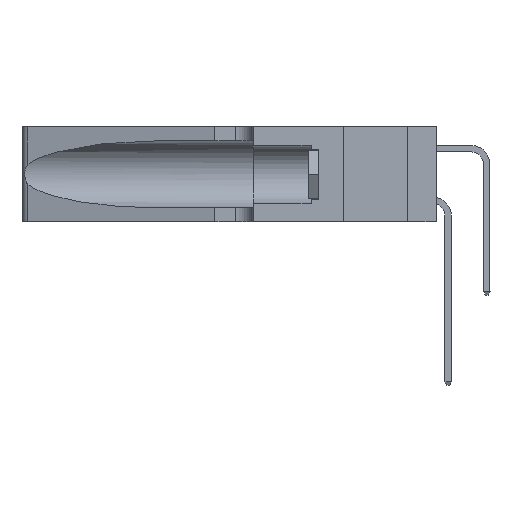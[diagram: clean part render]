
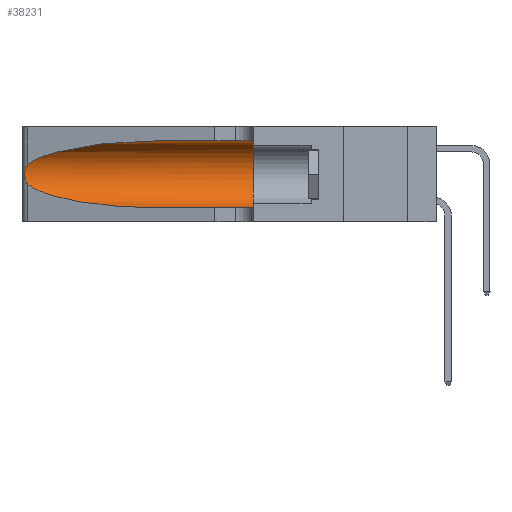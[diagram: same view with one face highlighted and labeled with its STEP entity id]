
A CAD part, left-side view. The second image highlights one B-rep face of the part: STEP entity #38231.
In plain terms, the highlighted cylindrical face has radius 3.308 mm (diameter 6.617 mm), a partial arc.
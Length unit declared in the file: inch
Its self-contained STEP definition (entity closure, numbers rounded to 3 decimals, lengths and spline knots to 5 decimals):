
#231 = CARTESIAN_POINT ( 'NONE',  ( 0.25639, 1.23184, 0.21858 ) ) ;
#267 = CIRCLE ( 'NONE', #12914, 0.13025 ) ;
#367 = CARTESIAN_POINT ( 'NONE',  ( 0.25639, 1.23186, 0.15144 ) ) ;
#790 = CARTESIAN_POINT ( 'NONE',  ( 0.1305, 0.35, 0.05475 ) ) ;
#2662 = CARTESIAN_POINT ( 'NONE',  ( 0.25487, 1.22718, 0.22369 ) ) ;
#3551 = DIRECTION ( 'NONE',  ( 0., -1., 0. ) ) ;
#3570 = CARTESIAN_POINT ( 'NONE',  ( 0.25487, 1.22718, 0.14631 ) ) ;
#3775 = EDGE_CURVE ( 'NONE', #7832, #8609, #11327, .T. ) ;
#4247 =( BOUNDED_CURVE ( )  B_SPLINE_CURVE ( 3, ( #21486, #18471, #12590, #33351 ),
 .UNSPECIFIED., .F., .T. ) 
 B_SPLINE_CURVE_WITH_KNOTS ( ( 4, 4 ),
 ( 1.5708, 2.84003 ),
 .UNSPECIFIED. ) 
 CURVE ( )  GEOMETRIC_REPRESENTATION_ITEM ( )  RATIONAL_B_SPLINE_CURVE ( ( 1., 0.87, 0.87, 1. ) ) 
 REPRESENTATION_ITEM ( '' )  );
#4338 = CARTESIAN_POINT ( 'NONE',  ( 0.1305, 0.72297, 0.31525 ) ) ;
#4430 = EDGE_CURVE ( 'NONE', #9524, #7832, #4247, .T. ) ;
#4561 = VECTOR ( 'NONE', #3551, 39.37008 ) ;
#4654 = EDGE_CURVE ( 'NONE', #17662, #17156, #267, .T. ) ;
#4661 = EDGE_CURVE ( 'NONE', #8609, #13584, #36060, .T. ) ;
#6535 = EDGE_CURVE ( 'NONE', #9524, #17662, #12644, .T. ) ;
#7121 = ORIENTED_EDGE ( 'NONE', *, *, #4430, .T. ) ;
#7679 = CARTESIAN_POINT ( 'NONE',  ( 0.18966, 0.96281, 0.05475 ) ) ;
#7735 = CARTESIAN_POINT ( 'NONE',  ( 0.1305, 1.61858, 0.185 ) ) ;
#7832 = VERTEX_POINT ( 'NONE', #2662 ) ;
#8125 = DIRECTION ( 'NONE',  ( 0., -1., 0. ) ) ;
#8609 = VERTEX_POINT ( 'NONE', #36108 ) ;
#9524 = VERTEX_POINT ( 'NONE', #4338 ) ;
#9611 = CARTESIAN_POINT ( 'NONE',  ( 0.25854, 1.2359, 0.20912 ) ) ;
#10641 = VECTOR ( 'NONE', #8125, 39.37008 ) ;
#10675 = ORIENTED_EDGE ( 'NONE', *, *, #4654, .F. ) ;
#11327 = B_SPLINE_CURVE_WITH_KNOTS ( 'NONE', 3,
 ( #24488, #21532, #231, #27455, #9611, #30449, #12633, #33399, #15659, #36359, #18641, #367, #21673, #3570 ),
 .UNSPECIFIED., .F., .F.,
 ( 4, 2, 2, 2, 2, 2, 4 ),
 ( 0., 0.00027, 0.00053, 0.00107, 0.0016, 0.00187, 0.00214 ),
 .UNSPECIFIED. ) ;
#12033 = ORIENTED_EDGE ( 'NONE', *, *, #19330, .T. ) ;
#12590 = CARTESIAN_POINT ( 'NONE',  ( 0.2373, 1.15595, 0.28018 ) ) ;
#12633 = CARTESIAN_POINT ( 'NONE',  ( 0.26075, 1.23896, 0.19203 ) ) ;
#12644 = LINE ( 'NONE', #27562, #4561 ) ;
#12677 = FACE_OUTER_BOUND ( 'NONE', #28007, .T. ) ;
#12914 = AXIS2_PLACEMENT_3D ( 'NONE', #34375, #16666, #37336 ) ;
#13584 = VERTEX_POINT ( 'NONE', #20951 ) ;
#15659 = CARTESIAN_POINT ( 'NONE',  ( 0.26017, 1.23833, 0.17102 ) ) ;
#16666 = DIRECTION ( 'NONE',  ( 0., 1., 0. ) ) ;
#17156 = VERTEX_POINT ( 'NONE', #790 ) ;
#17662 = VERTEX_POINT ( 'NONE', #30029 ) ;
#18471 = CARTESIAN_POINT ( 'NONE',  ( 0.18966, 0.96281, 0.31525 ) ) ;
#18641 = CARTESIAN_POINT ( 'NONE',  ( 0.25789, 1.23486, 0.15765 ) ) ;
#19330 = EDGE_CURVE ( 'NONE', #13584, #17156, #36172, .T. ) ;
#19654 = CARTESIAN_POINT ( 'NONE',  ( 0.25487, 1.22718, 0.14631 ) ) ;
#19716 = DIRECTION ( 'NONE',  ( 0., -1., 0. ) ) ;
#20536 = ORIENTED_EDGE ( 'NONE', *, *, #6535, .F. ) ;
#20951 = CARTESIAN_POINT ( 'NONE',  ( 0.1305, 0.72297, 0.05475 ) ) ;
#21486 = CARTESIAN_POINT ( 'NONE',  ( 0.1305, 0.72297, 0.31525 ) ) ;
#21532 = CARTESIAN_POINT ( 'NONE',  ( 0.25555, 1.22994, 0.2215 ) ) ;
#21673 = CARTESIAN_POINT ( 'NONE',  ( 0.25555, 1.22993, 0.14849 ) ) ;
#22647 = CARTESIAN_POINT ( 'NONE',  ( 0.2373, 1.15595, 0.08982 ) ) ;
#24361 = AXIS2_PLACEMENT_3D ( 'NONE', #7735, #19716, #28611 ) ;
#24488 = CARTESIAN_POINT ( 'NONE',  ( 0.25487, 1.22718, 0.22369 ) ) ;
#25110 = ORIENTED_EDGE ( 'NONE', *, *, #4661, .T. ) ;
#26028 = CARTESIAN_POINT ( 'NONE',  ( 0.1305, 1.61858, 0.05475 ) ) ;
#27455 = CARTESIAN_POINT ( 'NONE',  ( 0.25787, 1.23484, 0.2124 ) ) ;
#27562 = CARTESIAN_POINT ( 'NONE',  ( 0.1305, 1.61858, 0.31525 ) ) ;
#28007 = EDGE_LOOP ( 'NONE', ( #7121, #38009, #25110, #12033, #10675, #20536 ) ) ;
#28553 = CARTESIAN_POINT ( 'NONE',  ( 0.1305, 0.72297, 0.05475 ) ) ;
#28611 = DIRECTION ( 'NONE',  ( 0., 0., -1. ) ) ;
#30029 = CARTESIAN_POINT ( 'NONE',  ( 0.1305, 0.35, 0.31525 ) ) ;
#30449 = CARTESIAN_POINT ( 'NONE',  ( 0.26018, 1.23835, 0.19895 ) ) ;
#33351 = CARTESIAN_POINT ( 'NONE',  ( 0.25487, 1.22718, 0.22369 ) ) ;
#33399 = CARTESIAN_POINT ( 'NONE',  ( 0.26075, 1.23896, 0.178 ) ) ;
#34375 = CARTESIAN_POINT ( 'NONE',  ( 0.1305, 0.35, 0.185 ) ) ;
#35409 = CYLINDRICAL_SURFACE ( 'NONE', #24361, 0.13025 ) ;
#36060 =( BOUNDED_CURVE ( )  B_SPLINE_CURVE ( 3, ( #19654, #22647, #7679, #28553 ),
 .UNSPECIFIED., .F., .T. ) 
 B_SPLINE_CURVE_WITH_KNOTS ( ( 4, 4 ),
 ( 3.44316, 4.71239 ),
 .UNSPECIFIED. ) 
 CURVE ( )  GEOMETRIC_REPRESENTATION_ITEM ( )  RATIONAL_B_SPLINE_CURVE ( ( 1., 0.87, 0.87, 1. ) ) 
 REPRESENTATION_ITEM ( '' )  );
#36108 = CARTESIAN_POINT ( 'NONE',  ( 0.25487, 1.22718, 0.14631 ) ) ;
#36172 = LINE ( 'NONE', #26028, #10641 ) ;
#36359 = CARTESIAN_POINT ( 'NONE',  ( 0.25856, 1.23593, 0.16098 ) ) ;
#37336 = DIRECTION ( 'NONE',  ( 0., 0., 1. ) ) ;
#38009 = ORIENTED_EDGE ( 'NONE', *, *, #3775, .T. ) ;
#38231 = ADVANCED_FACE ( 'NONE', ( #12677 ), #35409, .F. ) ;
